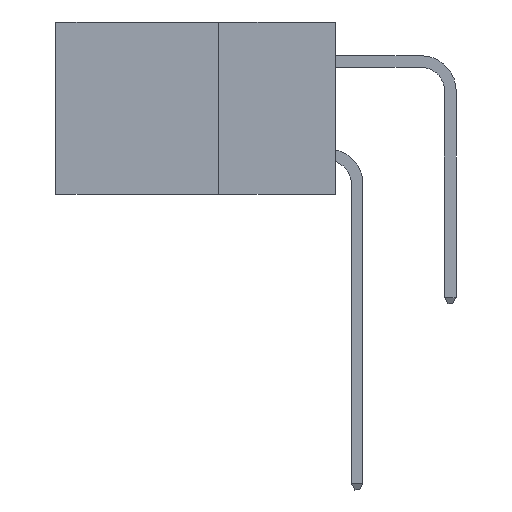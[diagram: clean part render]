
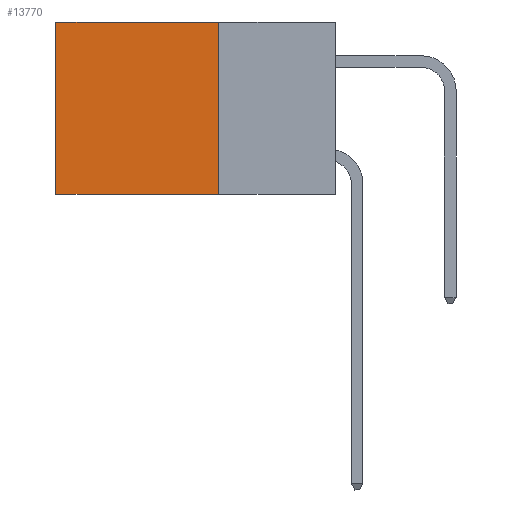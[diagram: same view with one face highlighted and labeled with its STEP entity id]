
A CAD part, left-side view. The second image highlights one B-rep face of the part: STEP entity #13770.
In plain terms, the highlighted planar face has unit normal (-1, 0, 0).
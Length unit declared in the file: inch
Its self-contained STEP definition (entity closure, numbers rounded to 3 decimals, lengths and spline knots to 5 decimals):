
#270 = ORIENTED_EDGE ( 'NONE', *, *, #12908, .F. ) ;
#546 = EDGE_CURVE ( 'NONE', #555, #9655, #9834, .T. ) ;
#555 = VERTEX_POINT ( 'NONE', #11713 ) ;
#1514 = DIRECTION ( 'NONE',  ( 0., 0., -1. ) ) ;
#1857 = CARTESIAN_POINT ( 'NONE',  ( 0.2875, 0.6, -0.37 ) ) ;
#1923 = CARTESIAN_POINT ( 'NONE',  ( 0.2875, 0.25, 0. ) ) ;
#2994 = CARTESIAN_POINT ( 'NONE',  ( 0.2875, 0.25, -0.37 ) ) ;
#3501 = PLANE ( 'NONE',  #11661 ) ;
#3653 = ORIENTED_EDGE ( 'NONE', *, *, #546, .F. ) ;
#4615 = CARTESIAN_POINT ( 'NONE',  ( 0.2875, 0.25, 0. ) ) ;
#4967 = ORIENTED_EDGE ( 'NONE', *, *, #14004, .T. ) ;
#5138 = LINE ( 'NONE', #10520, #13958 ) ;
#5701 = DIRECTION ( 'NONE',  ( 1., 0., 0. ) ) ;
#7150 = CARTESIAN_POINT ( 'NONE',  ( 0.2875, 0.6, 0. ) ) ;
#7722 = EDGE_CURVE ( 'NONE', #555, #9138, #12486, .T. ) ;
#7903 = CARTESIAN_POINT ( 'NONE',  ( 0.2875, 0.25, 0. ) ) ;
#8217 = CARTESIAN_POINT ( 'NONE',  ( 0.2875, 0.25, -0.37 ) ) ;
#9138 = VERTEX_POINT ( 'NONE', #7150 ) ;
#9332 = ORIENTED_EDGE ( 'NONE', *, *, #7722, .T. ) ;
#9577 = VECTOR ( 'NONE', #11219, 39.37008 ) ;
#9655 = VERTEX_POINT ( 'NONE', #8217 ) ;
#9834 = LINE ( 'NONE', #1923, #13427 ) ;
#10187 = LINE ( 'NONE', #2994, #12603 ) ;
#10520 = CARTESIAN_POINT ( 'NONE',  ( 0.2875, 0.6, 0. ) ) ;
#10740 = DIRECTION ( 'NONE',  ( 0., 1., 0. ) ) ;
#11087 = VERTEX_POINT ( 'NONE', #1857 ) ;
#11219 = DIRECTION ( 'NONE',  ( 0., 1., 0. ) ) ;
#11622 = DIRECTION ( 'NONE',  ( 0., 0., -1. ) ) ;
#11661 = AXIS2_PLACEMENT_3D ( 'NONE', #4615, #5701, #13443 ) ;
#11713 = CARTESIAN_POINT ( 'NONE',  ( 0.2875, 0.25, 0. ) ) ;
#11788 = EDGE_LOOP ( 'NONE', ( #4967, #270, #3653, #9332 ) ) ;
#12486 = LINE ( 'NONE', #7903, #9577 ) ;
#12603 = VECTOR ( 'NONE', #10740, 39.37008 ) ;
#12908 = EDGE_CURVE ( 'NONE', #9655, #11087, #10187, .T. ) ;
#13427 = VECTOR ( 'NONE', #1514, 39.37008 ) ;
#13443 = DIRECTION ( 'NONE',  ( 0., 0., -1. ) ) ;
#13770 = ADVANCED_FACE ( 'NONE', ( #13795 ), #3501, .F. ) ;
#13795 = FACE_OUTER_BOUND ( 'NONE', #11788, .T. ) ;
#13958 = VECTOR ( 'NONE', #11622, 39.37008 ) ;
#14004 = EDGE_CURVE ( 'NONE', #9138, #11087, #5138, .T. ) ;
